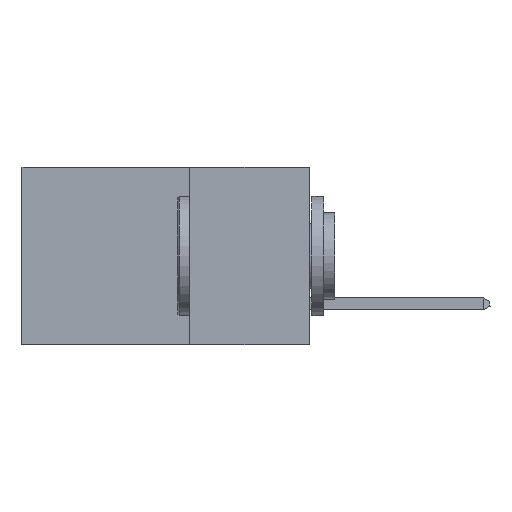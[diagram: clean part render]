
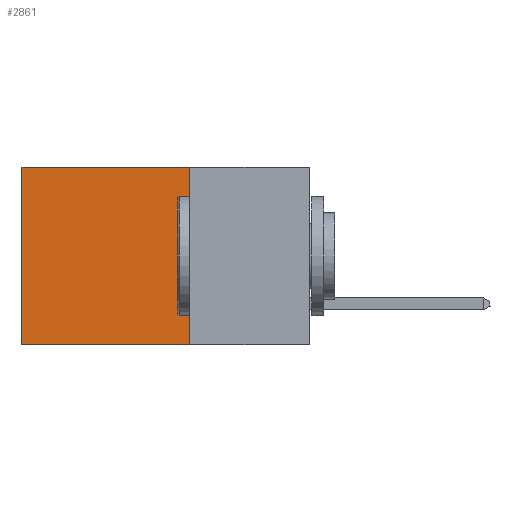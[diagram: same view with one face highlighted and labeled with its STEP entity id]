
A CAD part, left-side view. The second image highlights one B-rep face of the part: STEP entity #2861.
In plain terms, the highlighted planar face has unit normal (-1, 0, 0).
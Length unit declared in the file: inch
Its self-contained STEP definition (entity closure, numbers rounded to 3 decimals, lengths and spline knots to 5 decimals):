
#37 = EDGE_CURVE ( 'NONE', #10959, #21417, #9399, .T. ) ;
#810 = ORIENTED_EDGE ( 'NONE', *, *, #37, .F. ) ;
#2738 = DIRECTION ( 'NONE',  ( 0., 1., 0. ) ) ;
#2752 = CARTESIAN_POINT ( 'NONE',  ( 0.2875, 0.6, 0. ) ) ;
#2861 = ADVANCED_FACE ( 'NONE', ( #10085 ), #21412, .F. ) ;
#3372 = VERTEX_POINT ( 'NONE', #26205 ) ;
#3498 = CARTESIAN_POINT ( 'NONE',  ( 0.2875, 0.25, 0. ) ) ;
#3876 = EDGE_CURVE ( 'NONE', #21721, #3372, #13095, .T. ) ;
#8523 = DIRECTION ( 'NONE',  ( 1., 0., 0. ) ) ;
#9399 = LINE ( 'NONE', #15384, #26655 ) ;
#9670 = ORIENTED_EDGE ( 'NONE', *, *, #24220, .F. ) ;
#10085 = FACE_OUTER_BOUND ( 'NONE', #25452, .T. ) ;
#10268 = CARTESIAN_POINT ( 'NONE',  ( 0.2875, 0.25, -0.37 ) ) ;
#10959 = VERTEX_POINT ( 'NONE', #10268 ) ;
#12612 = LINE ( 'NONE', #2752, #22016 ) ;
#13095 = LINE ( 'NONE', #17784, #22206 ) ;
#13532 = AXIS2_PLACEMENT_3D ( 'NONE', #21510, #8523, #23655 ) ;
#13563 = DIRECTION ( 'NONE',  ( 0., 1., 0. ) ) ;
#15384 = CARTESIAN_POINT ( 'NONE',  ( 0.2875, 0.25, -0.37 ) ) ;
#15956 = ORIENTED_EDGE ( 'NONE', *, *, #16627, .T. ) ;
#16627 = EDGE_CURVE ( 'NONE', #3372, #21417, #12612, .T. ) ;
#17308 = CARTESIAN_POINT ( 'NONE',  ( 0.2875, 0.6, -0.37 ) ) ;
#17784 = CARTESIAN_POINT ( 'NONE',  ( 0.2875, 0.25, 0. ) ) ;
#19714 = DIRECTION ( 'NONE',  ( 0., 0., -1. ) ) ;
#21412 = PLANE ( 'NONE',  #13532 ) ;
#21417 = VERTEX_POINT ( 'NONE', #17308 ) ;
#21510 = CARTESIAN_POINT ( 'NONE',  ( 0.2875, 0.25, 0. ) ) ;
#21721 = VERTEX_POINT ( 'NONE', #3498 ) ;
#22016 = VECTOR ( 'NONE', #23984, 39.37008 ) ;
#22153 = LINE ( 'NONE', #26142, #22851 ) ;
#22206 = VECTOR ( 'NONE', #13563, 39.37008 ) ;
#22851 = VECTOR ( 'NONE', #19714, 39.37008 ) ;
#23655 = DIRECTION ( 'NONE',  ( 0., 0., -1. ) ) ;
#23984 = DIRECTION ( 'NONE',  ( 0., 0., -1. ) ) ;
#24220 = EDGE_CURVE ( 'NONE', #21721, #10959, #22153, .T. ) ;
#25452 = EDGE_LOOP ( 'NONE', ( #15956, #810, #9670, #26258 ) ) ;
#26142 = CARTESIAN_POINT ( 'NONE',  ( 0.2875, 0.25, 0. ) ) ;
#26205 = CARTESIAN_POINT ( 'NONE',  ( 0.2875, 0.6, 0. ) ) ;
#26258 = ORIENTED_EDGE ( 'NONE', *, *, #3876, .T. ) ;
#26655 = VECTOR ( 'NONE', #2738, 39.37008 ) ;
